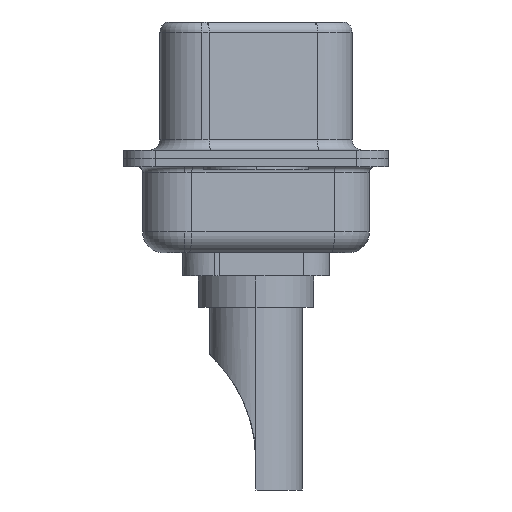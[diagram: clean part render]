
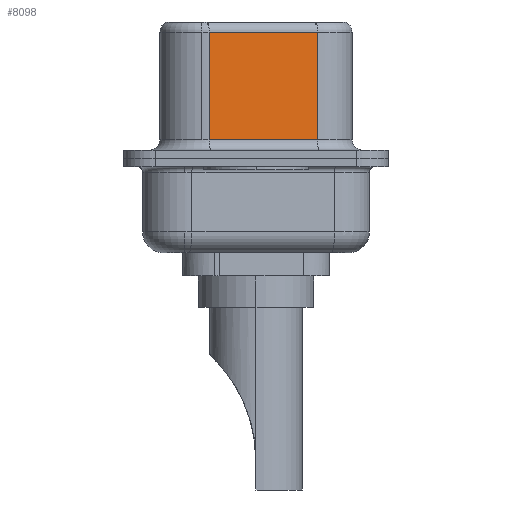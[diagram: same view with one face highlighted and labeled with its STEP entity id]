
A CAD part, left-side view. The second image highlights one B-rep face of the part: STEP entity #8098.
In plain terms, the highlighted planar face has unit normal (-0.985, -0.174, 0).
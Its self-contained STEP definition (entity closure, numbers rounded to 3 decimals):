
#1019 = DIRECTION ( 'NONE',  ( -0.174, 0.985, 0. ) ) ;
#1052 = LINE ( 'NONE', #10365, #13052 ) ;
#2330 = VECTOR ( 'NONE', #3270, 1000. ) ;
#2570 = ORIENTED_EDGE ( 'NONE', *, *, #5466, .F. ) ;
#3009 = DIRECTION ( 'NONE',  ( 0., 0., -1. ) ) ;
#3270 = DIRECTION ( 'NONE',  ( 0.174, -0.985, 0. ) ) ;
#3359 = EDGE_CURVE ( 'NONE', #10836, #10933, #6585, .T. ) ;
#4244 = CARTESIAN_POINT ( 'NONE',  ( 4.58, -2.927, 6.52 ) ) ;
#4997 = CARTESIAN_POINT ( 'NONE',  ( 3.67, 2.233, 0.9 ) ) ;
#5197 = VECTOR ( 'NONE', #3009, 1000. ) ;
#5466 = EDGE_CURVE ( 'NONE', #16291, #10933, #9358, .T. ) ;
#6585 = LINE ( 'NONE', #9378, #2330 ) ;
#6788 = ORIENTED_EDGE ( 'NONE', *, *, #8660, .T. ) ;
#7403 = CARTESIAN_POINT ( 'NONE',  ( 3.67, 2.233, 6.02 ) ) ;
#7417 = FACE_OUTER_BOUND ( 'NONE', #15130, .T. ) ;
#7463 = DIRECTION ( 'NONE',  ( -0.174, 0.985, 0. ) ) ;
#8098 = ADVANCED_FACE ( 'NONE', ( #7417 ), #8971, .F. ) ;
#8403 = CARTESIAN_POINT ( 'NONE',  ( 4.58, -2.927, 0.9 ) ) ;
#8660 = EDGE_CURVE ( 'NONE', #18555, #10836, #1052, .T. ) ;
#8662 = ORIENTED_EDGE ( 'NONE', *, *, #3359, .T. ) ;
#8971 = PLANE ( 'NONE',  #14966 ) ;
#9358 = LINE ( 'NONE', #4244, #5197 ) ;
#9378 = CARTESIAN_POINT ( 'NONE',  ( 4.58, -2.927, 0.9 ) ) ;
#10145 = VECTOR ( 'NONE', #7463, 1000. ) ;
#10365 = CARTESIAN_POINT ( 'NONE',  ( 3.67, 2.233, 6.52 ) ) ;
#10521 = DIRECTION ( 'NONE',  ( 0.985, 0.174, 0. ) ) ;
#10836 = VERTEX_POINT ( 'NONE', #4997 ) ;
#10933 = VERTEX_POINT ( 'NONE', #8403 ) ;
#11223 = EDGE_CURVE ( 'NONE', #16291, #18555, #18129, .T. ) ;
#13052 = VECTOR ( 'NONE', #17869, 1000. ) ;
#14851 = ORIENTED_EDGE ( 'NONE', *, *, #11223, .T. ) ;
#14966 = AXIS2_PLACEMENT_3D ( 'NONE', #19460, #10521, #1019 ) ;
#15130 = EDGE_LOOP ( 'NONE', ( #2570, #14851, #6788, #8662 ) ) ;
#16248 = CARTESIAN_POINT ( 'NONE',  ( 4.58, -2.927, 6.02 ) ) ;
#16291 = VERTEX_POINT ( 'NONE', #16248 ) ;
#17869 = DIRECTION ( 'NONE',  ( 0., 0., -1. ) ) ;
#18011 = CARTESIAN_POINT ( 'NONE',  ( 4.58, -2.927, 6.02 ) ) ;
#18129 = LINE ( 'NONE', #18011, #10145 ) ;
#18555 = VERTEX_POINT ( 'NONE', #7403 ) ;
#19460 = CARTESIAN_POINT ( 'NONE',  ( 4.58, -2.927, 6.52 ) ) ;
